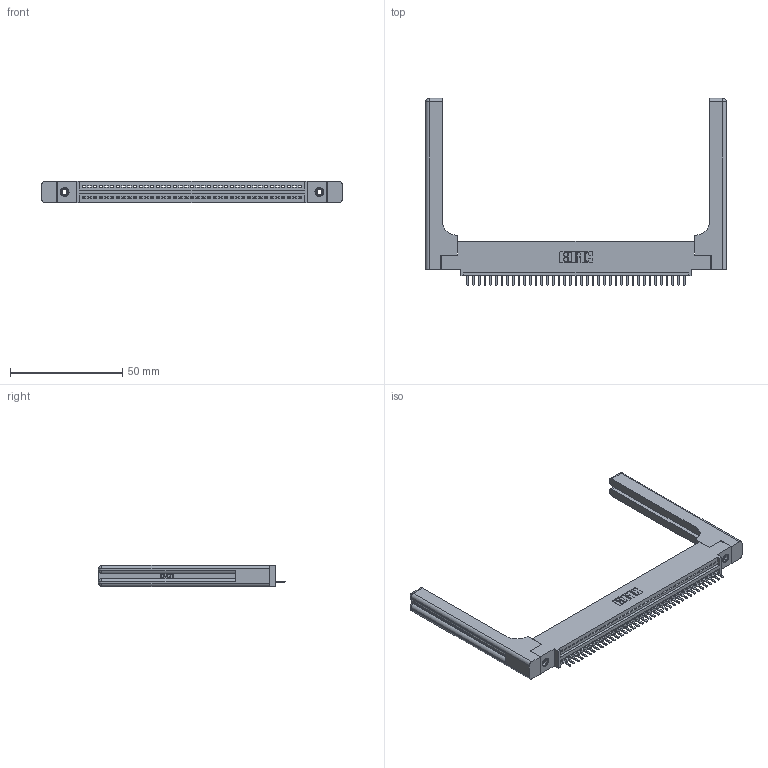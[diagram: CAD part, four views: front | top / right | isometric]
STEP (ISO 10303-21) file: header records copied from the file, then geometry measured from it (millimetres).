
FILE_DESCRIPTION (( 'STEP AP203' ), '1' );
FILE_NAME ('395-039-520-458.STEP', '2019-10-22T02:17:20', ( '' ), ( '' ), 'SwSTEP 2.0', 'SolidWorks 2016', '' );
FILE_SCHEMA (( 'CONFIG_CONTROL_DESIGN' ));
Length unit declared in the file: inch
Products named in the file (5): 345 Part_0.110 Offset - 0.156 Dia-TH; 345-250-001_345-250-001-102; 345-292-001_345-293-120; 395-039-520-458; 345-220-058_345-220-058
Assembly tree (44 placements, depth 2):
  395-039-520-458
    345 Part_0.110 Offset - 0.156 Dia-TH
    345-292-001_345-293-120  x39
    345-250-001_345-250-001-102  x2
    345-220-058_345-220-058  x2
Bounding box: 134.09 x 83.44 x 9.4 mm (x, y, z)
Volume: 21030.5 mm3; surface area: 21625 mm2
Topology: 44 solids, 44 shells, 2804 faces, 8195 edges, 5338 vertices
Faces by surface type: plane 1870, cylinder 874, bspline 36, cone 12, sphere 8, torus 4
Entity records: 35184 total; most frequent: CARTESIAN_POINT 7078, ORIENTED_EDGE 5836, DIRECTION 5120, EDGE_CURVE 2918, LINE 2534, VECTOR 2534, VERTEX_POINT 1934, AXIS2_PLACEMENT_3D 1293
